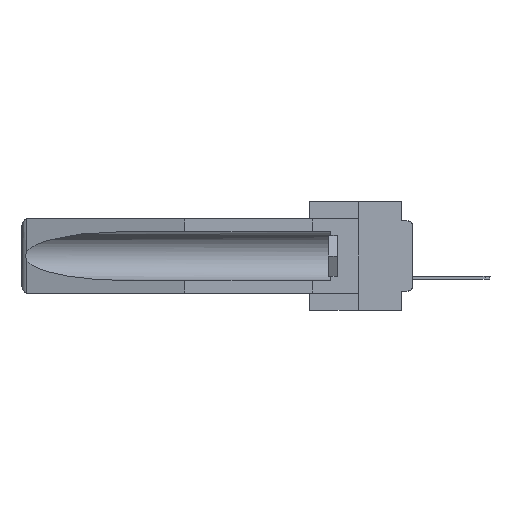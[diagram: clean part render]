
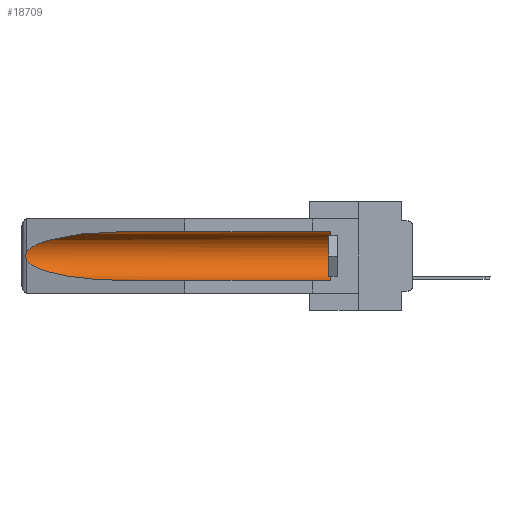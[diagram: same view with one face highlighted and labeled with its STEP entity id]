
A CAD part, left-side view. The second image highlights one B-rep face of the part: STEP entity #18709.
In plain terms, the highlighted cylindrical face has radius 2.857 mm (diameter 5.715 mm), a partial arc.
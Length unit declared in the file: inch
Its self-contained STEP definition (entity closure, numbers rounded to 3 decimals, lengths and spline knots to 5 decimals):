
#762 = CARTESIAN_POINT ( 'NONE',  ( 0.155, -0.30754, -0.059 ) ) ;
#1129 = CARTESIAN_POINT ( 'NONE',  ( 0.155, -0.30754, -0.284 ) ) ;
#1263 = DIRECTION ( 'NONE',  ( 0., -1., 0. ) ) ;
#1271 = VERTEX_POINT ( 'NONE', #13856 ) ;
#1859 = DIRECTION ( 'NONE',  ( 0., 0., 1. ) ) ;
#1943 = CARTESIAN_POINT ( 'NONE',  ( 0.26537, 1.52718, -0.19328 ) ) ;
#2714 = VERTEX_POINT ( 'NONE', #21212 ) ;
#2822 = LINE ( 'NONE', #762, #13898 ) ;
#3492 = EDGE_LOOP ( 'NONE', ( #3688, #27592, #15091, #4260, #4292, #4194 ) ) ;
#3688 = ORIENTED_EDGE ( 'NONE', *, *, #13667, .T. ) ;
#3767 = FACE_OUTER_BOUND ( 'NONE', #3492, .T. ) ;
#3850 = CARTESIAN_POINT ( 'NONE',  ( 0.25451, 1.48313, -0.24835 ) ) ;
#3899 = CYLINDRICAL_SURFACE ( 'NONE', #4418, 0.1125 ) ;
#4194 = ORIENTED_EDGE ( 'NONE', *, *, #27047, .T. ) ;
#4260 = ORIENTED_EDGE ( 'NONE', *, *, #21158, .F. ) ;
#4292 = ORIENTED_EDGE ( 'NONE', *, *, #19957, .T. ) ;
#4304 =( BOUNDED_CURVE ( )  B_SPLINE_CURVE ( 3, ( #1943, #3850, #12621, #21546 ),
 .UNSPECIFIED., .F., .T. ) 
 B_SPLINE_CURVE_WITH_KNOTS ( ( 4, 4 ),
 ( 0.1948, 1.5708 ),
 .UNSPECIFIED. ) 
 CURVE ( )  GEOMETRIC_REPRESENTATION_ITEM ( )  RATIONAL_B_SPLINE_CURVE ( ( 1., 0.848, 0.848, 1. ) ) 
 REPRESENTATION_ITEM ( '' )  );
#4418 = AXIS2_PLACEMENT_3D ( 'NONE', #25675, #7847, #5670 ) ;
#5670 = DIRECTION ( 'NONE',  ( 0., 0., 1. ) ) ;
#6396 = B_SPLINE_CURVE_WITH_KNOTS ( 'NONE', 3,
 ( #26430, #21795, #26733, #15207, #15077, #13167, #24096, #6723, #9053, #21950 ),
 .UNSPECIFIED., .F., .F.,
 ( 4, 2, 2, 2, 4 ),
 ( 0., 0.00029, 0.00058, 0.00087, 0.00117 ),
 .UNSPECIFIED. ) ;
#6554 = VERTEX_POINT ( 'NONE', #20608 ) ;
#6723 = CARTESIAN_POINT ( 'NONE',  ( 0.26655, 1.53094, -0.18657 ) ) ;
#7847 = DIRECTION ( 'NONE',  ( 0., 1., 0. ) ) ;
#9015 = EDGE_CURVE ( 'NONE', #11821, #18987, #4304, .T. ) ;
#9053 = CARTESIAN_POINT ( 'NONE',  ( 0.26597, 1.5296, -0.19026 ) ) ;
#10693 = AXIS2_PLACEMENT_3D ( 'NONE', #10775, #1263, #1859 ) ;
#10775 = CARTESIAN_POINT ( 'NONE',  ( 0.155, 0.126, -0.1715 ) ) ;
#11128 = CARTESIAN_POINT ( 'NONE',  ( 0.155, 1.07973, -0.059 ) ) ;
#11821 = VERTEX_POINT ( 'NONE', #18923 ) ;
#11864 = CARTESIAN_POINT ( 'NONE',  ( 0.155, 1.07973, -0.284 ) ) ;
#12151 = VECTOR ( 'NONE', #16371, 39.37008 ) ;
#12621 = CARTESIAN_POINT ( 'NONE',  ( 0.21114, 1.30732, -0.284 ) ) ;
#13167 = CARTESIAN_POINT ( 'NONE',  ( 0.2675, 1.53308, -0.17534 ) ) ;
#13667 = EDGE_CURVE ( 'NONE', #1271, #6554, #18140, .T. ) ;
#13856 = CARTESIAN_POINT ( 'NONE',  ( 0.155, 1.07973, -0.059 ) ) ;
#13898 = VECTOR ( 'NONE', #13920, 39.37008 ) ;
#13920 = DIRECTION ( 'NONE',  ( 0., 1., 0. ) ) ;
#15077 = CARTESIAN_POINT ( 'NONE',  ( 0.2675, 1.53308, -0.16763 ) ) ;
#15091 = ORIENTED_EDGE ( 'NONE', *, *, #9015, .T. ) ;
#15207 = CARTESIAN_POINT ( 'NONE',  ( 0.2673, 1.5327, -0.16383 ) ) ;
#16371 = DIRECTION ( 'NONE',  ( 0., 1., 0. ) ) ;
#17561 = CARTESIAN_POINT ( 'NONE',  ( 0.25451, 1.48313, -0.09465 ) ) ;
#18016 = VERTEX_POINT ( 'NONE', #28756 ) ;
#18140 =( BOUNDED_CURVE ( )  B_SPLINE_CURVE ( 3, ( #11128, #24702, #17561, #26450 ),
 .UNSPECIFIED., .F., .T. ) 
 B_SPLINE_CURVE_WITH_KNOTS ( ( 4, 4 ),
 ( 4.71239, 6.08839 ),
 .UNSPECIFIED. ) 
 CURVE ( )  GEOMETRIC_REPRESENTATION_ITEM ( )  RATIONAL_B_SPLINE_CURVE ( ( 1., 0.848, 0.848, 1. ) ) 
 REPRESENTATION_ITEM ( '' )  );
#18709 = ADVANCED_FACE ( 'NONE', ( #3767 ), #3899, .F. ) ;
#18923 = CARTESIAN_POINT ( 'NONE',  ( 0.26537, 1.52718, -0.19328 ) ) ;
#18987 = VERTEX_POINT ( 'NONE', #11864 ) ;
#19957 = EDGE_CURVE ( 'NONE', #18016, #2714, #26076, .T. ) ;
#20608 = CARTESIAN_POINT ( 'NONE',  ( 0.26537, 1.52718, -0.14972 ) ) ;
#21158 = EDGE_CURVE ( 'NONE', #18016, #18987, #21175, .T. ) ;
#21175 = LINE ( 'NONE', #1129, #12151 ) ;
#21212 = CARTESIAN_POINT ( 'NONE',  ( 0.155, 0.126, -0.059 ) ) ;
#21546 = CARTESIAN_POINT ( 'NONE',  ( 0.155, 1.07973, -0.284 ) ) ;
#21795 = CARTESIAN_POINT ( 'NONE',  ( 0.26597, 1.52961, -0.15275 ) ) ;
#21950 = CARTESIAN_POINT ( 'NONE',  ( 0.26537, 1.52718, -0.19328 ) ) ;
#23949 = EDGE_CURVE ( 'NONE', #6554, #11821, #6396, .T. ) ;
#24096 = CARTESIAN_POINT ( 'NONE',  ( 0.2673, 1.53269, -0.17917 ) ) ;
#24702 = CARTESIAN_POINT ( 'NONE',  ( 0.21114, 1.30732, -0.059 ) ) ;
#25675 = CARTESIAN_POINT ( 'NONE',  ( 0.155, -0.30754, -0.1715 ) ) ;
#26076 = CIRCLE ( 'NONE', #10693, 0.1125 ) ;
#26430 = CARTESIAN_POINT ( 'NONE',  ( 0.26537, 1.52718, -0.14972 ) ) ;
#26450 = CARTESIAN_POINT ( 'NONE',  ( 0.26537, 1.52718, -0.14972 ) ) ;
#26733 = CARTESIAN_POINT ( 'NONE',  ( 0.26654, 1.53092, -0.15636 ) ) ;
#27047 = EDGE_CURVE ( 'NONE', #2714, #1271, #2822, .T. ) ;
#27592 = ORIENTED_EDGE ( 'NONE', *, *, #23949, .T. ) ;
#28756 = CARTESIAN_POINT ( 'NONE',  ( 0.155, 0.126, -0.284 ) ) ;
